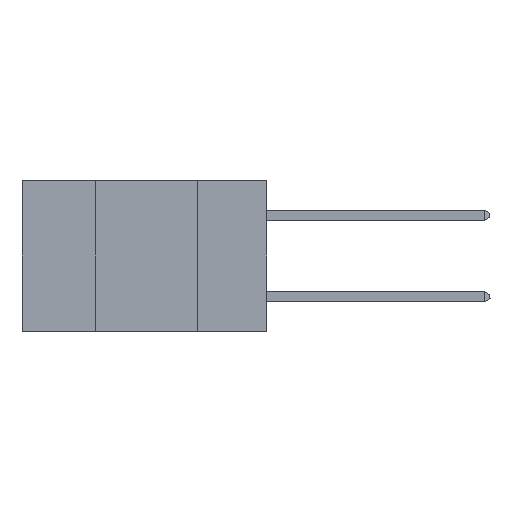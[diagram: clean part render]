
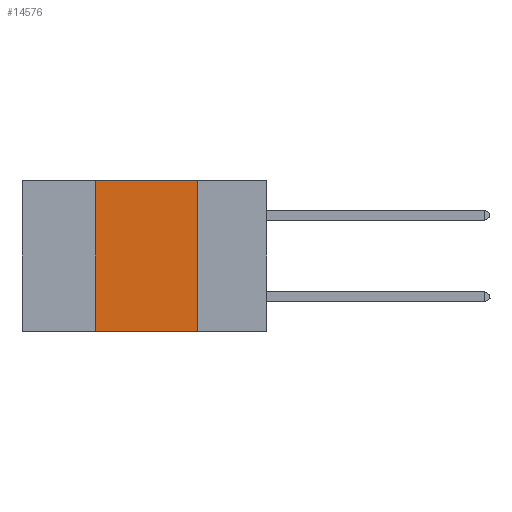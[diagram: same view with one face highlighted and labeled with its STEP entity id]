
A CAD part, left-side view. The second image highlights one B-rep face of the part: STEP entity #14576.
In plain terms, the highlighted planar face has unit normal (-1, 0, 0).
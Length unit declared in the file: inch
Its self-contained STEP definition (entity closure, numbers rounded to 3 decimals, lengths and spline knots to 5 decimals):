
#284 = CARTESIAN_POINT ( 'NONE',  ( 0., 0.6, 0. ) ) ;
#1234 = DIRECTION ( 'NONE',  ( 0., 0., -1. ) ) ;
#1829 = DIRECTION ( 'NONE',  ( 1., 0., 0. ) ) ;
#1976 = VERTEX_POINT ( 'NONE', #13506 ) ;
#2040 = CARTESIAN_POINT ( 'NONE',  ( 0., 0.42, 0. ) ) ;
#2723 = VERTEX_POINT ( 'NONE', #18703 ) ;
#3203 = EDGE_CURVE ( 'NONE', #4825, #6032, #17649, .T. ) ;
#3338 = VECTOR ( 'NONE', #3604, 39.37008 ) ;
#3604 = DIRECTION ( 'NONE',  ( 0., 0., 1. ) ) ;
#4825 = VERTEX_POINT ( 'NONE', #9841 ) ;
#5178 = VECTOR ( 'NONE', #1234, 39.37008 ) ;
#5489 = DIRECTION ( 'NONE',  ( 0., -1., 0. ) ) ;
#5747 = AXIS2_PLACEMENT_3D ( 'NONE', #284, #1829, #12345 ) ;
#6032 = VERTEX_POINT ( 'NONE', #11019 ) ;
#6917 = EDGE_CURVE ( 'NONE', #1976, #2723, #7010, .T. ) ;
#7010 = LINE ( 'NONE', #8473, #18485 ) ;
#8473 = CARTESIAN_POINT ( 'NONE',  ( 0., 0.6, -0.37 ) ) ;
#8702 = VECTOR ( 'NONE', #17593, 39.37008 ) ;
#9841 = CARTESIAN_POINT ( 'NONE',  ( 0., 0.42, 0. ) ) ;
#10226 = CARTESIAN_POINT ( 'NONE',  ( 0., 0.17, 0. ) ) ;
#10816 = PLANE ( 'NONE',  #5747 ) ;
#11019 = CARTESIAN_POINT ( 'NONE',  ( 0., 0.17, 0. ) ) ;
#12264 = ORIENTED_EDGE ( 'NONE', *, *, #16936, .F. ) ;
#12345 = DIRECTION ( 'NONE',  ( 0., 0., -1. ) ) ;
#12658 = ORIENTED_EDGE ( 'NONE', *, *, #3203, .F. ) ;
#13157 = ORIENTED_EDGE ( 'NONE', *, *, #17251, .F. ) ;
#13506 = CARTESIAN_POINT ( 'NONE',  ( 0., 0.42, -0.37 ) ) ;
#13979 = EDGE_LOOP ( 'NONE', ( #13157, #12658, #12264, #18179 ) ) ;
#14576 = ADVANCED_FACE ( 'NONE', ( #17883 ), #10816, .F. ) ;
#15776 = LINE ( 'NONE', #2040, #3338 ) ;
#16681 = LINE ( 'NONE', #10226, #5178 ) ;
#16936 = EDGE_CURVE ( 'NONE', #1976, #4825, #15776, .T. ) ;
#17251 = EDGE_CURVE ( 'NONE', #6032, #2723, #16681, .T. ) ;
#17593 = DIRECTION ( 'NONE',  ( 0., -1., 0. ) ) ;
#17649 = LINE ( 'NONE', #17986, #8702 ) ;
#17883 = FACE_OUTER_BOUND ( 'NONE', #13979, .T. ) ;
#17986 = CARTESIAN_POINT ( 'NONE',  ( 0., 0.6, 0. ) ) ;
#18179 = ORIENTED_EDGE ( 'NONE', *, *, #6917, .T. ) ;
#18485 = VECTOR ( 'NONE', #5489, 39.37008 ) ;
#18703 = CARTESIAN_POINT ( 'NONE',  ( 0., 0.17, -0.37 ) ) ;
